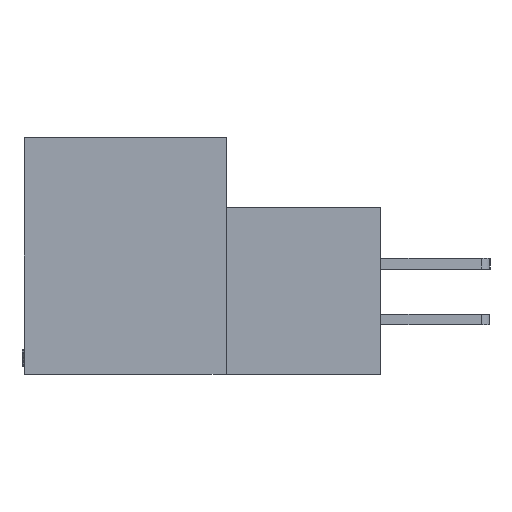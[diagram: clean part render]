
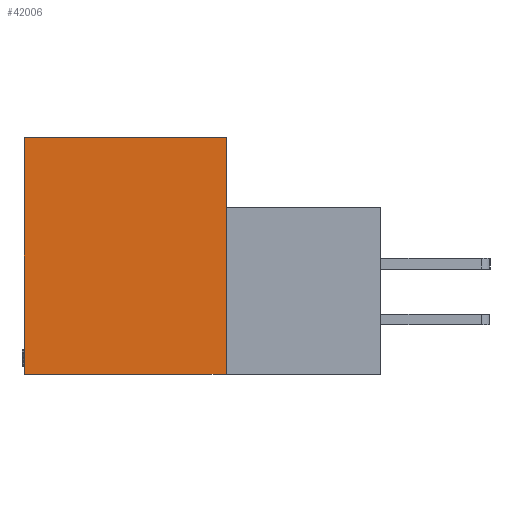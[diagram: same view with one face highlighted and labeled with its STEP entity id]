
A CAD part, left-side view. The second image highlights one B-rep face of the part: STEP entity #42006.
In plain terms, the highlighted planar face has unit normal (-1, 0, 0).
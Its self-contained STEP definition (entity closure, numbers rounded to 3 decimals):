
#100 = CARTESIAN_POINT ( 'NONE',  ( 0., 11.506, -13.487 ) ) ;
#1041 = LINE ( 'NONE', #38984, #37571 ) ;
#3736 = CARTESIAN_POINT ( 'NONE',  ( 0., 11.506, -13.487 ) ) ;
#5292 = DIRECTION ( 'NONE',  ( 0., -1., 0. ) ) ;
#5398 = DIRECTION ( 'NONE',  ( 0., 0., -1. ) ) ;
#6986 = ORIENTED_EDGE ( 'NONE', *, *, #12515, .F. ) ;
#8252 = EDGE_CURVE ( 'NONE', #14832, #22020, #43425, .T. ) ;
#10942 = PLANE ( 'NONE',  #44194 ) ;
#12515 = EDGE_CURVE ( 'NONE', #22020, #15778, #1041, .T. ) ;
#14176 = CARTESIAN_POINT ( 'NONE',  ( 0., 0., -13.487 ) ) ;
#14533 = DIRECTION ( 'NONE',  ( 1., 0., 0. ) ) ;
#14832 = VERTEX_POINT ( 'NONE', #39790 ) ;
#14873 = DIRECTION ( 'NONE',  ( 0., 1., 0. ) ) ;
#15778 = VERTEX_POINT ( 'NONE', #100 ) ;
#16090 = CARTESIAN_POINT ( 'NONE',  ( 0., 0., 0. ) ) ;
#17789 = CARTESIAN_POINT ( 'NONE',  ( 0., 0., 0. ) ) ;
#18195 = LINE ( 'NONE', #26490, #31415 ) ;
#21661 = DIRECTION ( 'NONE',  ( 0., 0., -1. ) ) ;
#22020 = VERTEX_POINT ( 'NONE', #14176 ) ;
#25981 = EDGE_LOOP ( 'NONE', ( #6986, #34472, #40259, #28261 ) ) ;
#26490 = CARTESIAN_POINT ( 'NONE',  ( 0., 11.506, 0. ) ) ;
#26866 = EDGE_CURVE ( 'NONE', #39507, #14832, #18195, .T. ) ;
#28261 = ORIENTED_EDGE ( 'NONE', *, *, #45243, .F. ) ;
#29172 = FACE_OUTER_BOUND ( 'NONE', #25981, .T. ) ;
#31415 = VECTOR ( 'NONE', #5292, 1000. ) ;
#31904 = CARTESIAN_POINT ( 'NONE',  ( 0., 11.506, 0. ) ) ;
#34472 = ORIENTED_EDGE ( 'NONE', *, *, #8252, .F. ) ;
#35751 = LINE ( 'NONE', #3736, #37435 ) ;
#37435 = VECTOR ( 'NONE', #45835, 1000. ) ;
#37571 = VECTOR ( 'NONE', #14873, 1000. ) ;
#38984 = CARTESIAN_POINT ( 'NONE',  ( 0., -8.814, -13.487 ) ) ;
#39507 = VERTEX_POINT ( 'NONE', #31904 ) ;
#39790 = CARTESIAN_POINT ( 'NONE',  ( 0., 0., 0. ) ) ;
#40259 = ORIENTED_EDGE ( 'NONE', *, *, #26866, .F. ) ;
#42006 = ADVANCED_FACE ( 'NONE', ( #29172 ), #10942, .F. ) ;
#43425 = LINE ( 'NONE', #16090, #43958 ) ;
#43958 = VECTOR ( 'NONE', #5398, 1000. ) ;
#44194 = AXIS2_PLACEMENT_3D ( 'NONE', #17789, #14533, #21661 ) ;
#45243 = EDGE_CURVE ( 'NONE', #15778, #39507, #35751, .T. ) ;
#45835 = DIRECTION ( 'NONE',  ( 0., 0., 1. ) ) ;
